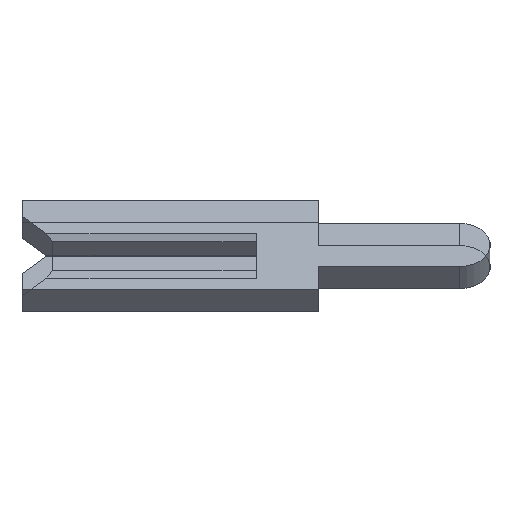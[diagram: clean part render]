
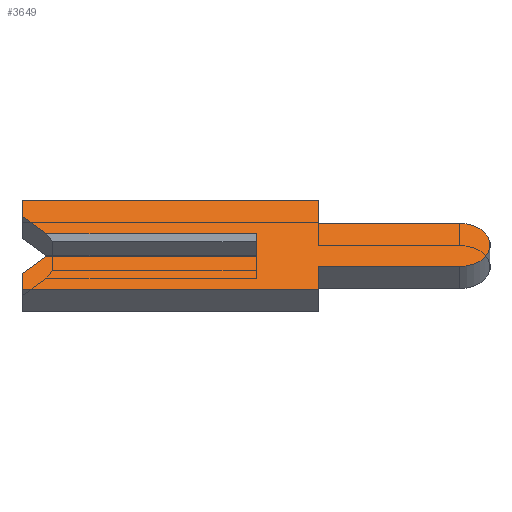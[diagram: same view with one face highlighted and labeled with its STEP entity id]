
A CAD part, left-side view. The second image highlights one B-rep face of the part: STEP entity #3649.
In plain terms, the highlighted face is planar.
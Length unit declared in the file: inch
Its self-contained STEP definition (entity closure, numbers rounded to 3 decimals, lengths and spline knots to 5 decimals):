
#6 = LINE ( 'NONE', #4175, #2606 ) ;
#89 = CIRCLE ( 'NONE', #989, 0.0195 ) ;
#150 = VERTEX_POINT ( 'NONE', #3596 ) ;
#257 = DIRECTION ( 'NONE',  ( 0., 0.707, 0.707 ) ) ;
#334 = ORIENTED_EDGE ( 'NONE', *, *, #3330, .F. ) ;
#372 = ORIENTED_EDGE ( 'NONE', *, *, #636, .F. ) ;
#373 = DIRECTION ( 'NONE',  ( 0., 1., 0. ) ) ;
#467 = CARTESIAN_POINT ( 'NONE',  ( -0.01, -0.1305, 0.0195 ) ) ;
#601 = DIRECTION ( 'NONE',  ( 0., 0., -1. ) ) ;
#615 = EDGE_CURVE ( 'NONE', #1631, #1669, #1955, .T. ) ;
#636 = EDGE_CURVE ( 'NONE', #2756, #3835, #2778, .T. ) ;
#653 = EDGE_LOOP ( 'NONE', ( #2479, #2459, #4306, #3106, #1021, #692, #2828, #372, #4362, #2732, #3707, #2861, #1292, #334 ) ) ;
#656 = VECTOR ( 'NONE', #1341, 39.37008 ) ;
#692 = ORIENTED_EDGE ( 'NONE', *, *, #2485, .F. ) ;
#792 = DIRECTION ( 'NONE',  ( 0., 0., -1. ) ) ;
#867 = CARTESIAN_POINT ( 'NONE',  ( -0.01, 0., 0.0065 ) ) ;
#891 = EDGE_CURVE ( 'NONE', #2080, #1891, #1479, .T. ) ;
#989 = AXIS2_PLACEMENT_3D ( 'NONE', #991, #4617, #601 ) ;
#991 = CARTESIAN_POINT ( 'NONE',  ( -0.01, -0.1305, 0. ) ) ;
#1008 = LINE ( 'NONE', #867, #3522 ) ;
#1021 = ORIENTED_EDGE ( 'NONE', *, *, #2867, .F. ) ;
#1196 = LINE ( 'NONE', #2082, #4111 ) ;
#1202 = DIRECTION ( 'NONE',  ( 0., -1., 0. ) ) ;
#1292 = ORIENTED_EDGE ( 'NONE', *, *, #3396, .F. ) ;
#1311 = VECTOR ( 'NONE', #4213, 39.37008 ) ;
#1318 = DIRECTION ( 'NONE',  ( 0., 0., 1. ) ) ;
#1341 = DIRECTION ( 'NONE',  ( 0., 0., 1. ) ) ;
#1346 = VERTEX_POINT ( 'NONE', #2291 ) ;
#1379 = CARTESIAN_POINT ( 'NONE',  ( -0.01, -0.04, -0.04 ) ) ;
#1432 = DIRECTION ( 'NONE',  ( 1., 0., 0. ) ) ;
#1472 = LINE ( 'NONE', #2010, #2221 ) ;
#1479 = LINE ( 'NONE', #3334, #3744 ) ;
#1519 = LINE ( 'NONE', #1903, #3053 ) ;
#1523 = DIRECTION ( 'NONE',  ( 0., 0., -1. ) ) ;
#1553 = CARTESIAN_POINT ( 'NONE',  ( -0.01, 0., 0.01 ) ) ;
#1621 = CARTESIAN_POINT ( 'NONE',  ( -0.01, -0.1305, -0.0195 ) ) ;
#1631 = VERTEX_POINT ( 'NONE', #2618 ) ;
#1669 = VERTEX_POINT ( 'NONE', #4496 ) ;
#1703 = EDGE_CURVE ( 'NONE', #4332, #2317, #2401, .T. ) ;
#1769 = VECTOR ( 'NONE', #1202, 39.37008 ) ;
#1832 = VECTOR ( 'NONE', #373, 39.37008 ) ;
#1873 = VECTOR ( 'NONE', #3673, 39.37008 ) ;
#1891 = VERTEX_POINT ( 'NONE', #4427 ) ;
#1903 = CARTESIAN_POINT ( 'NONE',  ( -0.01, -0.04, 0.04 ) ) ;
#1912 = FACE_OUTER_BOUND ( 'NONE', #653, .T. ) ;
#1955 = LINE ( 'NONE', #2923, #1873 ) ;
#2005 = LINE ( 'NONE', #1379, #1311 ) ;
#2010 = CARTESIAN_POINT ( 'NONE',  ( -0.01, 0.15, -0.026 ) ) ;
#2043 = DIRECTION ( 'NONE',  ( 0., 1., 0. ) ) ;
#2080 = VERTEX_POINT ( 'NONE', #3382 ) ;
#2082 = CARTESIAN_POINT ( 'NONE',  ( -0.01, 0.15, 0.01 ) ) ;
#2169 = PLANE ( 'NONE',  #3579 ) ;
#2219 = VECTOR ( 'NONE', #257, 39.37008 ) ;
#2221 = VECTOR ( 'NONE', #1318, 39.37008 ) ;
#2222 = CARTESIAN_POINT ( 'NONE',  ( -0.01, -0.04, -0.0195 ) ) ;
#2252 = EDGE_CURVE ( 'NONE', #1891, #2357, #1008, .T. ) ;
#2291 = CARTESIAN_POINT ( 'NONE',  ( -0.01, 0.15, 0.026 ) ) ;
#2317 = VERTEX_POINT ( 'NONE', #467 ) ;
#2339 = CARTESIAN_POINT ( 'NONE',  ( -0.01, -0.04, 0.0195 ) ) ;
#2357 = VERTEX_POINT ( 'NONE', #1553 ) ;
#2401 = LINE ( 'NONE', #2339, #1769 ) ;
#2459 = ORIENTED_EDGE ( 'NONE', *, *, #2252, .F. ) ;
#2479 = ORIENTED_EDGE ( 'NONE', *, *, #3138, .T. ) ;
#2485 = EDGE_CURVE ( 'NONE', #4482, #2582, #6, .T. ) ;
#2508 = DIRECTION ( 'NONE',  ( 0., -0.707, 0.707 ) ) ;
#2581 = DIRECTION ( 'NONE',  ( 0., -1., 0. ) ) ;
#2582 = VERTEX_POINT ( 'NONE', #3778 ) ;
#2595 = CARTESIAN_POINT ( 'NONE',  ( -0.01, 0.1305, -0.0065 ) ) ;
#2606 = VECTOR ( 'NONE', #2043, 39.37008 ) ;
#2618 = CARTESIAN_POINT ( 'NONE',  ( -0.01, 0.15, 0.04 ) ) ;
#2717 = LINE ( 'NONE', #3532, #2219 ) ;
#2732 = ORIENTED_EDGE ( 'NONE', *, *, #1703, .F. ) ;
#2756 = VERTEX_POINT ( 'NONE', #1621 ) ;
#2778 = LINE ( 'NONE', #2222, #1832 ) ;
#2822 = LINE ( 'NONE', #3505, #656 ) ;
#2828 = ORIENTED_EDGE ( 'NONE', *, *, #3571, .F. ) ;
#2858 = CARTESIAN_POINT ( 'NONE',  ( -0.01, -0.1305, 0. ) ) ;
#2861 = ORIENTED_EDGE ( 'NONE', *, *, #615, .F. ) ;
#2867 = EDGE_CURVE ( 'NONE', #2582, #150, #1472, .T. ) ;
#2923 = CARTESIAN_POINT ( 'NONE',  ( -0.01, 0.15, 0.04 ) ) ;
#2961 = CARTESIAN_POINT ( 'NONE',  ( -0.01, -0.04, -0.04 ) ) ;
#3053 = VECTOR ( 'NONE', #792, 39.37008 ) ;
#3071 = EDGE_CURVE ( 'NONE', #2317, #2756, #89, .T. ) ;
#3106 = ORIENTED_EDGE ( 'NONE', *, *, #4044, .F. ) ;
#3138 = EDGE_CURVE ( 'NONE', #4042, #2357, #1196, .T. ) ;
#3330 = EDGE_CURVE ( 'NONE', #4042, #1346, #2717, .T. ) ;
#3334 = CARTESIAN_POINT ( 'NONE',  ( -0.01, -0.1305, -0.01 ) ) ;
#3382 = CARTESIAN_POINT ( 'NONE',  ( -0.01, 0.134, -0.01 ) ) ;
#3396 = EDGE_CURVE ( 'NONE', #1346, #1631, #2822, .T. ) ;
#3469 = DIRECTION ( 'NONE',  ( 0., 0., 1. ) ) ;
#3505 = CARTESIAN_POINT ( 'NONE',  ( -0.01, 0.15, 0.026 ) ) ;
#3522 = VECTOR ( 'NONE', #3469, 39.37008 ) ;
#3532 = CARTESIAN_POINT ( 'NONE',  ( -0.01, 0.1305, 0.0065 ) ) ;
#3563 = CARTESIAN_POINT ( 'NONE',  ( -0.01, 0.134, 0.01 ) ) ;
#3571 = EDGE_CURVE ( 'NONE', #3835, #4482, #2005, .T. ) ;
#3579 = AXIS2_PLACEMENT_3D ( 'NONE', #2858, #1432, #1523 ) ;
#3596 = CARTESIAN_POINT ( 'NONE',  ( -0.01, 0.15, -0.026 ) ) ;
#3649 = ADVANCED_FACE ( 'NONE', ( #1912 ), #2169, .F. ) ;
#3661 = VECTOR ( 'NONE', #2508, 39.37008 ) ;
#3673 = DIRECTION ( 'NONE',  ( 0., -1., 0. ) ) ;
#3707 = ORIENTED_EDGE ( 'NONE', *, *, #4090, .F. ) ;
#3744 = VECTOR ( 'NONE', #2581, 39.37008 ) ;
#3778 = CARTESIAN_POINT ( 'NONE',  ( -0.01, 0.15, -0.04 ) ) ;
#3835 = VERTEX_POINT ( 'NONE', #4420 ) ;
#3913 = DIRECTION ( 'NONE',  ( 0., -1., 0. ) ) ;
#3926 = CARTESIAN_POINT ( 'NONE',  ( -0.01, -0.04, 0.0195 ) ) ;
#3948 = LINE ( 'NONE', #2595, #3661 ) ;
#4042 = VERTEX_POINT ( 'NONE', #3563 ) ;
#4044 = EDGE_CURVE ( 'NONE', #150, #2080, #3948, .T. ) ;
#4090 = EDGE_CURVE ( 'NONE', #1669, #4332, #1519, .T. ) ;
#4111 = VECTOR ( 'NONE', #3913, 39.37008 ) ;
#4175 = CARTESIAN_POINT ( 'NONE',  ( -0.01, 0.15, -0.04 ) ) ;
#4213 = DIRECTION ( 'NONE',  ( 0., 0., -1. ) ) ;
#4306 = ORIENTED_EDGE ( 'NONE', *, *, #891, .F. ) ;
#4332 = VERTEX_POINT ( 'NONE', #3926 ) ;
#4362 = ORIENTED_EDGE ( 'NONE', *, *, #3071, .F. ) ;
#4420 = CARTESIAN_POINT ( 'NONE',  ( -0.01, -0.04, -0.0195 ) ) ;
#4427 = CARTESIAN_POINT ( 'NONE',  ( -0.01, 0., -0.01 ) ) ;
#4482 = VERTEX_POINT ( 'NONE', #2961 ) ;
#4496 = CARTESIAN_POINT ( 'NONE',  ( -0.01, -0.04, 0.04 ) ) ;
#4617 = DIRECTION ( 'NONE',  ( 1., 0., 0. ) ) ;
